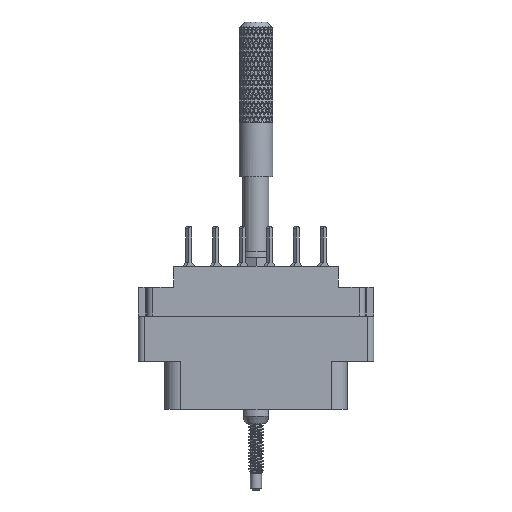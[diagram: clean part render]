
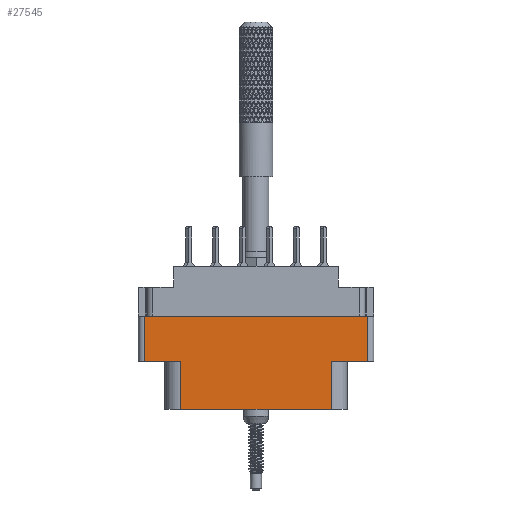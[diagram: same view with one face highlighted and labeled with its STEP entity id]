
A CAD part, front view. The second image highlights one B-rep face of the part: STEP entity #27545.
In plain terms, the highlighted planar face has unit normal (0, -1, 0).
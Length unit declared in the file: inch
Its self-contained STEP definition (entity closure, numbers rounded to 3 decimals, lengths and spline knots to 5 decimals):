
#1503 = DIRECTION ( 'NONE',  ( 0., 0., -1. ) ) ;
#1548 = CARTESIAN_POINT ( 'NONE',  ( -0.42, -0.343, -0.529 ) ) ;
#13404 = ORIENTED_EDGE ( 'NONE', *, *, #166642, .F. ) ;
#13662 = ORIENTED_EDGE ( 'NONE', *, *, #41978, .F. ) ;
#14473 = CARTESIAN_POINT ( 'NONE',  ( 0.42, -0.343, -0.529 ) ) ;
#20052 = VERTEX_POINT ( 'NONE', #155657 ) ;
#20252 = ORIENTED_EDGE ( 'NONE', *, *, #104979, .T. ) ;
#21183 = VERTEX_POINT ( 'NONE', #52113 ) ;
#22193 = LINE ( 'NONE', #132177, #117387 ) ;
#25722 = CARTESIAN_POINT ( 'NONE',  ( -0.42, -0.343, -0.529 ) ) ;
#27545 = ADVANCED_FACE ( 'NONE', ( #79191 ), #52188, .T. ) ;
#31368 = VERTEX_POINT ( 'NONE', #1548 ) ;
#34724 = DIRECTION ( 'NONE',  ( 0., 0., -1. ) ) ;
#37052 = LINE ( 'NONE', #89801, #167765 ) ;
#38243 = LINE ( 'NONE', #79395, #117995 ) ;
#41676 = EDGE_CURVE ( 'NONE', #83969, #31368, #38243, .T. ) ;
#41978 = EDGE_CURVE ( 'NONE', #21183, #112638, #120089, .T. ) ;
#45020 = CARTESIAN_POINT ( 'NONE',  ( 0.624, -0.343, -0.277 ) ) ;
#46088 = CARTESIAN_POINT ( 'NONE',  ( -0.624, -0.343, -0.798 ) ) ;
#48618 = DIRECTION ( 'NONE',  ( 1., 0., 0. ) ) ;
#48881 = CARTESIAN_POINT ( 'NONE',  ( 0., -0.343, -0.529 ) ) ;
#52113 = CARTESIAN_POINT ( 'NONE',  ( 0.624, -0.343, -0.529 ) ) ;
#52188 = PLANE ( 'NONE',  #56326 ) ;
#56326 = AXIS2_PLACEMENT_3D ( 'NONE', #151282, #135205, #121578 ) ;
#66299 = ORIENTED_EDGE ( 'NONE', *, *, #127312, .T. ) ;
#73852 = CARTESIAN_POINT ( 'NONE',  ( -0.42, -0.343, -0.798 ) ) ;
#76408 = VECTOR ( 'NONE', #172836, 39.37008 ) ;
#79191 = FACE_OUTER_BOUND ( 'NONE', #140632, .T. ) ;
#79395 = CARTESIAN_POINT ( 'NONE',  ( 0., -0.343, -0.529 ) ) ;
#80713 = CARTESIAN_POINT ( 'NONE',  ( -0.624, -0.343, -0.798 ) ) ;
#83969 = VERTEX_POINT ( 'NONE', #164243 ) ;
#85812 = LINE ( 'NONE', #46088, #119044 ) ;
#88663 = EDGE_CURVE ( 'NONE', #21183, #161197, #129461, .T. ) ;
#89504 = ORIENTED_EDGE ( 'NONE', *, *, #41676, .T. ) ;
#89801 = CARTESIAN_POINT ( 'NONE',  ( 0.42, -0.343, -0.529 ) ) ;
#93596 = DIRECTION ( 'NONE',  ( 1., 0., 0. ) ) ;
#95689 = VECTOR ( 'NONE', #153453, 39.37008 ) ;
#104979 = EDGE_CURVE ( 'NONE', #180496, #126086, #85812, .T. ) ;
#112638 = VERTEX_POINT ( 'NONE', #14473 ) ;
#115069 = ORIENTED_EDGE ( 'NONE', *, *, #159426, .F. ) ;
#117387 = VECTOR ( 'NONE', #48618, 39.37008 ) ;
#117995 = VECTOR ( 'NONE', #93596, 39.37008 ) ;
#118887 = ORIENTED_EDGE ( 'NONE', *, *, #171553, .F. ) ;
#119044 = VECTOR ( 'NONE', #160586, 39.37008 ) ;
#120089 = LINE ( 'NONE', #48881, #95689 ) ;
#121578 = DIRECTION ( 'NONE',  ( 0., 0., -1. ) ) ;
#126086 = VERTEX_POINT ( 'NONE', #154322 ) ;
#127312 = EDGE_CURVE ( 'NONE', #31368, #180496, #179680, .T. ) ;
#129461 = LINE ( 'NONE', #146181, #76408 ) ;
#131735 = VECTOR ( 'NONE', #165507, 39.37008 ) ;
#132177 = CARTESIAN_POINT ( 'NONE',  ( -0.656, -0.343, -0.277 ) ) ;
#135205 = DIRECTION ( 'NONE',  ( 0., -1., 0. ) ) ;
#140632 = EDGE_LOOP ( 'NONE', ( #66299, #20252, #13404, #13662, #140675, #115069, #118887, #89504 ) ) ;
#140675 = ORIENTED_EDGE ( 'NONE', *, *, #88663, .T. ) ;
#146181 = CARTESIAN_POINT ( 'NONE',  ( 0.624, -0.343, -0.798 ) ) ;
#151282 = CARTESIAN_POINT ( 'NONE',  ( -0.624, -0.343, -0.798 ) ) ;
#153453 = DIRECTION ( 'NONE',  ( -1., 0., 0. ) ) ;
#154322 = CARTESIAN_POINT ( 'NONE',  ( 0.42, -0.343, -0.798 ) ) ;
#155657 = CARTESIAN_POINT ( 'NONE',  ( -0.624, -0.343, -0.277 ) ) ;
#159426 = EDGE_CURVE ( 'NONE', #20052, #161197, #22193, .T. ) ;
#160586 = DIRECTION ( 'NONE',  ( 1., 0., 0. ) ) ;
#161197 = VERTEX_POINT ( 'NONE', #45020 ) ;
#164243 = CARTESIAN_POINT ( 'NONE',  ( -0.624, -0.343, -0.529 ) ) ;
#165507 = DIRECTION ( 'NONE',  ( 0., 0., 1. ) ) ;
#166642 = EDGE_CURVE ( 'NONE', #112638, #126086, #37052, .T. ) ;
#167765 = VECTOR ( 'NONE', #34724, 39.37008 ) ;
#171553 = EDGE_CURVE ( 'NONE', #83969, #20052, #180634, .T. ) ;
#172836 = DIRECTION ( 'NONE',  ( 0., 0., 1. ) ) ;
#173157 = VECTOR ( 'NONE', #1503, 39.37008 ) ;
#179680 = LINE ( 'NONE', #25722, #173157 ) ;
#180496 = VERTEX_POINT ( 'NONE', #73852 ) ;
#180634 = LINE ( 'NONE', #80713, #131735 ) ;
